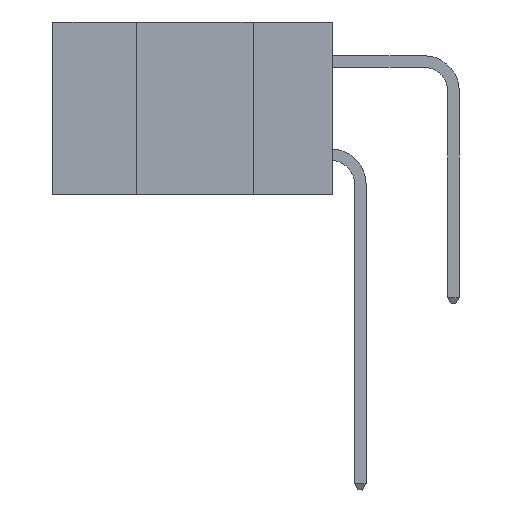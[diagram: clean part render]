
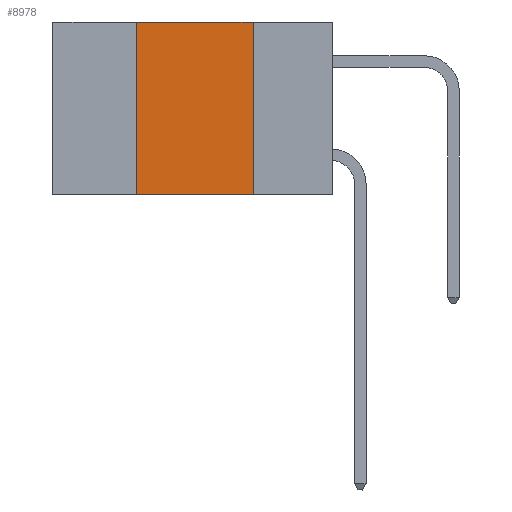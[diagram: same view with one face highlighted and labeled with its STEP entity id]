
A CAD part, left-side view. The second image highlights one B-rep face of the part: STEP entity #8978.
In plain terms, the highlighted planar face has unit normal (-1, 0, 0).
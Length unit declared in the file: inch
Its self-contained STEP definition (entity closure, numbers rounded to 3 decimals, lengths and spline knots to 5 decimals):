
#75 = VERTEX_POINT ( 'NONE', #12596 ) ;
#378 = VERTEX_POINT ( 'NONE', #2492 ) ;
#2143 = EDGE_CURVE ( 'NONE', #75, #7397, #9632, .T. ) ;
#2276 = EDGE_CURVE ( 'NONE', #7397, #378, #10365, .T. ) ;
#2492 = CARTESIAN_POINT ( 'NONE',  ( 0., 0.17, 0. ) ) ;
#3342 = VECTOR ( 'NONE', #9852, 39.37008 ) ;
#3583 = AXIS2_PLACEMENT_3D ( 'NONE', #9221, #12560, #6993 ) ;
#3659 = CARTESIAN_POINT ( 'NONE',  ( 0., 0.6, 0. ) ) ;
#3939 = CARTESIAN_POINT ( 'NONE',  ( 0., 0.17, -0.37 ) ) ;
#4082 = VERTEX_POINT ( 'NONE', #7891 ) ;
#5147 = CARTESIAN_POINT ( 'NONE',  ( 0., 0.42, 0. ) ) ;
#5443 = VECTOR ( 'NONE', #11786, 39.37008 ) ;
#6192 = ORIENTED_EDGE ( 'NONE', *, *, #2276, .F. ) ;
#6993 = DIRECTION ( 'NONE',  ( 0., 0., -1. ) ) ;
#7397 = VERTEX_POINT ( 'NONE', #5147 ) ;
#7891 = CARTESIAN_POINT ( 'NONE',  ( 0., 0.17, -0.37 ) ) ;
#8184 = EDGE_CURVE ( 'NONE', #378, #4082, #14134, .T. ) ;
#8978 = ADVANCED_FACE ( 'NONE', ( #9139 ), #13747, .F. ) ;
#9139 = FACE_OUTER_BOUND ( 'NONE', #11587, .T. ) ;
#9221 = CARTESIAN_POINT ( 'NONE',  ( 0., 0.6, 0. ) ) ;
#9579 = DIRECTION ( 'NONE',  ( 0., -1., 0. ) ) ;
#9632 = LINE ( 'NONE', #11943, #5443 ) ;
#9741 = CARTESIAN_POINT ( 'NONE',  ( 0., 0.6, -0.37 ) ) ;
#9852 = DIRECTION ( 'NONE',  ( 0., 0., -1. ) ) ;
#9872 = ORIENTED_EDGE ( 'NONE', *, *, #2143, .F. ) ;
#10332 = EDGE_CURVE ( 'NONE', #75, #4082, #10775, .T. ) ;
#10365 = LINE ( 'NONE', #3659, #13469 ) ;
#10435 = VECTOR ( 'NONE', #9579, 39.37008 ) ;
#10775 = LINE ( 'NONE', #9741, #10435 ) ;
#10993 = DIRECTION ( 'NONE',  ( 0., -1., 0. ) ) ;
#11587 = EDGE_LOOP ( 'NONE', ( #12923, #6192, #9872, #14170 ) ) ;
#11786 = DIRECTION ( 'NONE',  ( 0., 0., 1. ) ) ;
#11943 = CARTESIAN_POINT ( 'NONE',  ( 0., 0.42, -0.37 ) ) ;
#12560 = DIRECTION ( 'NONE',  ( 1., 0., 0. ) ) ;
#12596 = CARTESIAN_POINT ( 'NONE',  ( 0., 0.42, -0.37 ) ) ;
#12923 = ORIENTED_EDGE ( 'NONE', *, *, #8184, .F. ) ;
#13469 = VECTOR ( 'NONE', #10993, 39.37008 ) ;
#13747 = PLANE ( 'NONE',  #3583 ) ;
#14134 = LINE ( 'NONE', #3939, #3342 ) ;
#14170 = ORIENTED_EDGE ( 'NONE', *, *, #10332, .T. ) ;
